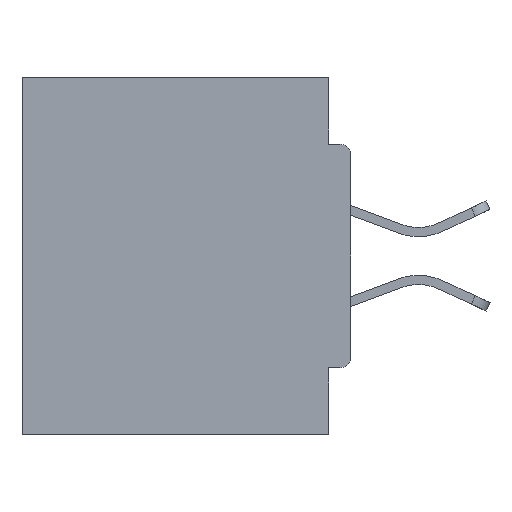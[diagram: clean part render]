
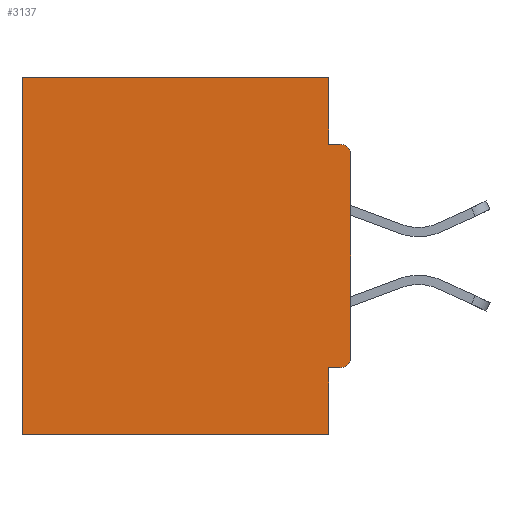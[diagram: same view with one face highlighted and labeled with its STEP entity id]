
A CAD part, left-side view. The second image highlights one B-rep face of the part: STEP entity #3137.
In plain terms, the highlighted planar face has unit normal (-1, 0, 0).
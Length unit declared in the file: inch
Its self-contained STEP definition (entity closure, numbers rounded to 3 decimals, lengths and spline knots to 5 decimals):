
#80 = ORIENTED_EDGE ( 'NONE', *, *, #8844, .F. ) ;
#134 = CARTESIAN_POINT ( 'NONE',  ( 0.298, 0.015, -0.3915 ) ) ;
#454 = CARTESIAN_POINT ( 'NONE',  ( 0.298, 0.46, 0. ) ) ;
#1273 = DIRECTION ( 'NONE',  ( 0., 1., 0. ) ) ;
#1892 = AXIS2_PLACEMENT_3D ( 'NONE', #20847, #5836, #25685 ) ;
#2278 = DIRECTION ( 'NONE',  ( -1., 0., 0. ) ) ;
#2568 = CARTESIAN_POINT ( 'NONE',  ( 0.298, 0.031, 0. ) ) ;
#2799 = CARTESIAN_POINT ( 'NONE',  ( 0.298, 0.46, 0. ) ) ;
#3137 = ADVANCED_FACE ( 'NONE', ( #9624 ), #7432, .F. ) ;
#3360 = VECTOR ( 'NONE', #10981, 39.37008 ) ;
#3746 = VECTOR ( 'NONE', #1273, 39.37008 ) ;
#3786 = CARTESIAN_POINT ( 'NONE',  ( 0.298, 0.031, -0.5 ) ) ;
#4232 = VECTOR ( 'NONE', #21509, 39.37008 ) ;
#4939 = VERTEX_POINT ( 'NONE', #6215 ) ;
#4974 = DIRECTION ( 'NONE',  ( 1., 0., 0. ) ) ;
#5218 = ORIENTED_EDGE ( 'NONE', *, *, #11869, .F. ) ;
#5285 = LINE ( 'NONE', #30950, #3746 ) ;
#5743 = CARTESIAN_POINT ( 'NONE',  ( 0.298, 0., -0.0935 ) ) ;
#5836 = DIRECTION ( 'NONE',  ( -1., 0., 0. ) ) ;
#5852 = VECTOR ( 'NONE', #15065, 39.37008 ) ;
#6215 = CARTESIAN_POINT ( 'NONE',  ( 0.298, 0., -0.3915 ) ) ;
#6442 = LINE ( 'NONE', #25691, #3360 ) ;
#6789 = VECTOR ( 'NONE', #20917, 39.37008 ) ;
#6819 = EDGE_CURVE ( 'NONE', #28540, #24168, #6442, .T. ) ;
#6847 = ORIENTED_EDGE ( 'NONE', *, *, #10139, .T. ) ;
#7432 = PLANE ( 'NONE',  #31335 ) ;
#7517 = EDGE_CURVE ( 'NONE', #17008, #18328, #28395, .T. ) ;
#8547 = VECTOR ( 'NONE', #14697, 39.37008 ) ;
#8634 = CARTESIAN_POINT ( 'NONE',  ( 0.298, 0., -0.5 ) ) ;
#8730 = ORIENTED_EDGE ( 'NONE', *, *, #14348, .T. ) ;
#8844 = EDGE_CURVE ( 'NONE', #24168, #27248, #30242, .T. ) ;
#8974 = EDGE_CURVE ( 'NONE', #16087, #9988, #14734, .T. ) ;
#9273 = VERTEX_POINT ( 'NONE', #29446 ) ;
#9610 = LINE ( 'NONE', #14445, #4232 ) ;
#9624 = FACE_OUTER_BOUND ( 'NONE', #25309, .T. ) ;
#9773 = EDGE_CURVE ( 'NONE', #17008, #4939, #11210, .T. ) ;
#9988 = VERTEX_POINT ( 'NONE', #22771 ) ;
#10139 = EDGE_CURVE ( 'NONE', #9273, #27248, #16198, .T. ) ;
#10153 = CARTESIAN_POINT ( 'NONE',  ( 0.298, 0.015, -0.4065 ) ) ;
#10981 = DIRECTION ( 'NONE',  ( 0., 0., -1. ) ) ;
#11210 = CIRCLE ( 'NONE', #29413, 0.015 ) ;
#11869 = EDGE_CURVE ( 'NONE', #18328, #16087, #21682, .T. ) ;
#13529 = CARTESIAN_POINT ( 'NONE',  ( 0.298, 0., -0.4065 ) ) ;
#14348 = EDGE_CURVE ( 'NONE', #28540, #17732, #5285, .T. ) ;
#14445 = CARTESIAN_POINT ( 'NONE',  ( 0.298, 0., 0. ) ) ;
#14697 = DIRECTION ( 'NONE',  ( 0., 0., -1. ) ) ;
#14734 = LINE ( 'NONE', #8634, #31373 ) ;
#14832 = ORIENTED_EDGE ( 'NONE', *, *, #6819, .F. ) ;
#14887 = ORIENTED_EDGE ( 'NONE', *, *, #7517, .F. ) ;
#15065 = DIRECTION ( 'NONE',  ( 0., 0., -1. ) ) ;
#15493 = ORIENTED_EDGE ( 'NONE', *, *, #20127, .F. ) ;
#16087 = VERTEX_POINT ( 'NONE', #3786 ) ;
#16198 = CIRCLE ( 'NONE', #1892, 0.015 ) ;
#16601 = CARTESIAN_POINT ( 'NONE',  ( 0.298, 0.031, -0.0935 ) ) ;
#17008 = VERTEX_POINT ( 'NONE', #10153 ) ;
#17009 = CARTESIAN_POINT ( 'NONE',  ( 0.298, 0., 0. ) ) ;
#17461 = DIRECTION ( 'NONE',  ( 0., 0., -1. ) ) ;
#17732 = VERTEX_POINT ( 'NONE', #2799 ) ;
#18328 = VERTEX_POINT ( 'NONE', #21004 ) ;
#18669 = DIRECTION ( 'NONE',  ( 0., 1., 0. ) ) ;
#18839 = EDGE_CURVE ( 'NONE', #17732, #9988, #22848, .T. ) ;
#20127 = EDGE_CURVE ( 'NONE', #9273, #4939, #9610, .T. ) ;
#20847 = CARTESIAN_POINT ( 'NONE',  ( 0.298, 0.015, -0.1085 ) ) ;
#20917 = DIRECTION ( 'NONE',  ( 0., 1., 0. ) ) ;
#21004 = CARTESIAN_POINT ( 'NONE',  ( 0.298, 0.031, -0.4065 ) ) ;
#21345 = VECTOR ( 'NONE', #25576, 39.37008 ) ;
#21509 = DIRECTION ( 'NONE',  ( 0., 0., -1. ) ) ;
#21682 = LINE ( 'NONE', #24661, #8547 ) ;
#22117 = CARTESIAN_POINT ( 'NONE',  ( 0.298, 0.015, -0.0935 ) ) ;
#22226 = DIRECTION ( 'NONE',  ( 0., 0., -1. ) ) ;
#22771 = CARTESIAN_POINT ( 'NONE',  ( 0.298, 0.46, -0.5 ) ) ;
#22848 = LINE ( 'NONE', #454, #5852 ) ;
#24168 = VERTEX_POINT ( 'NONE', #16601 ) ;
#24661 = CARTESIAN_POINT ( 'NONE',  ( 0.298, 0.031, -0.5 ) ) ;
#25277 = ORIENTED_EDGE ( 'NONE', *, *, #9773, .T. ) ;
#25309 = EDGE_LOOP ( 'NONE', ( #6847, #80, #14832, #8730, #25918, #29967, #5218, #14887, #25277, #15493 ) ) ;
#25576 = DIRECTION ( 'NONE',  ( 0., -1., 0. ) ) ;
#25685 = DIRECTION ( 'NONE',  ( 0., 0., -1. ) ) ;
#25691 = CARTESIAN_POINT ( 'NONE',  ( 0.298, 0.031, -0.5 ) ) ;
#25918 = ORIENTED_EDGE ( 'NONE', *, *, #18839, .T. ) ;
#27248 = VERTEX_POINT ( 'NONE', #22117 ) ;
#28395 = LINE ( 'NONE', #13529, #6789 ) ;
#28540 = VERTEX_POINT ( 'NONE', #2568 ) ;
#29413 = AXIS2_PLACEMENT_3D ( 'NONE', #134, #2278, #17461 ) ;
#29446 = CARTESIAN_POINT ( 'NONE',  ( 0.298, 0., -0.1085 ) ) ;
#29967 = ORIENTED_EDGE ( 'NONE', *, *, #8974, .F. ) ;
#30242 = LINE ( 'NONE', #5743, #21345 ) ;
#30950 = CARTESIAN_POINT ( 'NONE',  ( 0.298, 0., 0. ) ) ;
#31335 = AXIS2_PLACEMENT_3D ( 'NONE', #17009, #4974, #22226 ) ;
#31373 = VECTOR ( 'NONE', #18669, 39.37008 ) ;
